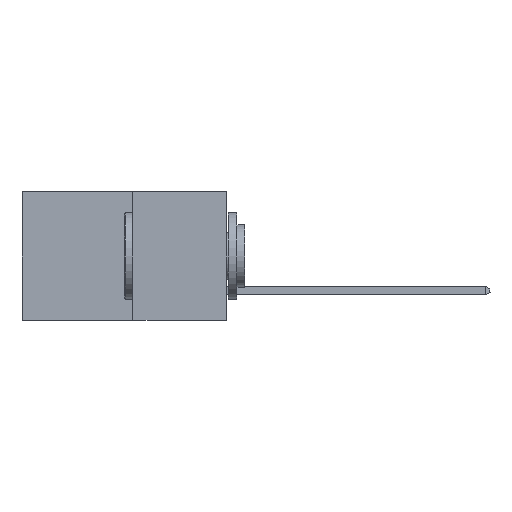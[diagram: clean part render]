
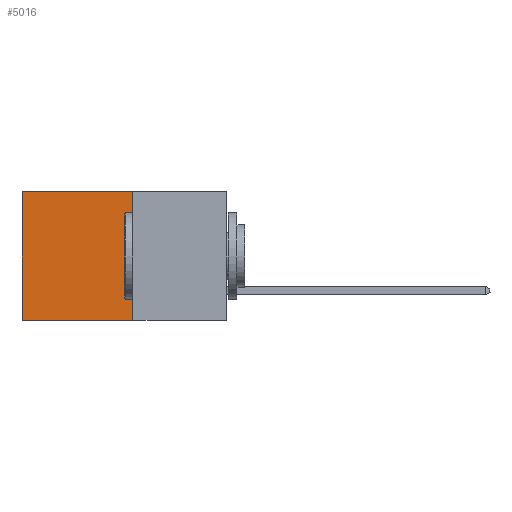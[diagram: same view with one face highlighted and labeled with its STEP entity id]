
A CAD part, left-side view. The second image highlights one B-rep face of the part: STEP entity #5016.
In plain terms, the highlighted planar face has unit normal (-1, 0, 0).
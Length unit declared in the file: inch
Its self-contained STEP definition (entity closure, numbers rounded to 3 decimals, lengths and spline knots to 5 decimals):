
#771 = ORIENTED_EDGE ( 'NONE', *, *, #15991, .F. ) ;
#1855 = EDGE_CURVE ( 'NONE', #7224, #7419, #12920, .T. ) ;
#1899 = CARTESIAN_POINT ( 'NONE',  ( 0.277, 0.27, 0. ) ) ;
#2595 = ORIENTED_EDGE ( 'NONE', *, *, #19718, .T. ) ;
#3286 = DIRECTION ( 'NONE',  ( 0., 0., -1. ) ) ;
#3312 = DIRECTION ( 'NONE',  ( 1., 0., 0. ) ) ;
#3427 = CARTESIAN_POINT ( 'NONE',  ( 0.277, 0.27, -0.37 ) ) ;
#3507 = PLANE ( 'NONE',  #15725 ) ;
#4298 = VECTOR ( 'NONE', #11633, 39.37008 ) ;
#5016 = ADVANCED_FACE ( 'NONE', ( #6484 ), #3507, .F. ) ;
#5355 = CARTESIAN_POINT ( 'NONE',  ( 0.277, 0.59, -0.37 ) ) ;
#5860 = DIRECTION ( 'NONE',  ( 0., 0., -1. ) ) ;
#6484 = FACE_OUTER_BOUND ( 'NONE', #8905, .T. ) ;
#6970 = DIRECTION ( 'NONE',  ( 0., 0., -1. ) ) ;
#7224 = VERTEX_POINT ( 'NONE', #18299 ) ;
#7419 = VERTEX_POINT ( 'NONE', #16738 ) ;
#8742 = DIRECTION ( 'NONE',  ( 0., 1., 0. ) ) ;
#8875 = LINE ( 'NONE', #9108, #16495 ) ;
#8905 = EDGE_LOOP ( 'NONE', ( #2595, #10316, #771, #20017 ) ) ;
#9108 = CARTESIAN_POINT ( 'NONE',  ( 0.277, 0.27, -0.37 ) ) ;
#10316 = ORIENTED_EDGE ( 'NONE', *, *, #1855, .F. ) ;
#11633 = DIRECTION ( 'NONE',  ( 0., 1., 0. ) ) ;
#12032 = LINE ( 'NONE', #5355, #20455 ) ;
#12044 = CARTESIAN_POINT ( 'NONE',  ( 0.277, 0.27, 0. ) ) ;
#12407 = CARTESIAN_POINT ( 'NONE',  ( 0.277, 0.27, -0.37 ) ) ;
#12920 = LINE ( 'NONE', #12407, #4298 ) ;
#13086 = VERTEX_POINT ( 'NONE', #1899 ) ;
#13281 = VECTOR ( 'NONE', #8742, 39.37008 ) ;
#13912 = EDGE_CURVE ( 'NONE', #13086, #15423, #17531, .T. ) ;
#15423 = VERTEX_POINT ( 'NONE', #18732 ) ;
#15725 = AXIS2_PLACEMENT_3D ( 'NONE', #3427, #3312, #3286 ) ;
#15991 = EDGE_CURVE ( 'NONE', #13086, #7224, #8875, .T. ) ;
#16495 = VECTOR ( 'NONE', #5860, 39.37008 ) ;
#16738 = CARTESIAN_POINT ( 'NONE',  ( 0.277, 0.59, -0.37 ) ) ;
#17531 = LINE ( 'NONE', #12044, #13281 ) ;
#18299 = CARTESIAN_POINT ( 'NONE',  ( 0.277, 0.27, -0.37 ) ) ;
#18732 = CARTESIAN_POINT ( 'NONE',  ( 0.277, 0.59, 0. ) ) ;
#19718 = EDGE_CURVE ( 'NONE', #15423, #7419, #12032, .T. ) ;
#20017 = ORIENTED_EDGE ( 'NONE', *, *, #13912, .T. ) ;
#20455 = VECTOR ( 'NONE', #6970, 39.37008 ) ;
